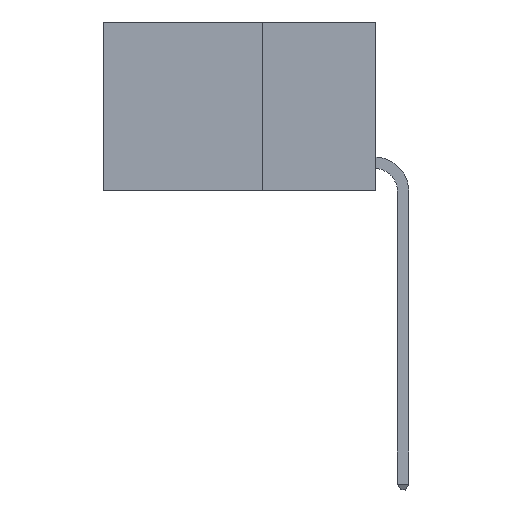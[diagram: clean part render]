
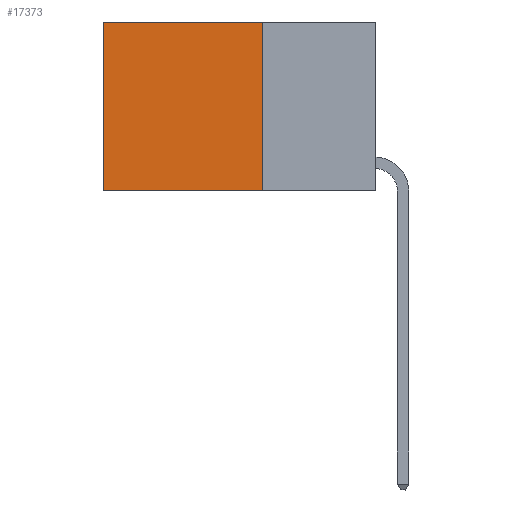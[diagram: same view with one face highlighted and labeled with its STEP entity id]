
A CAD part, left-side view. The second image highlights one B-rep face of the part: STEP entity #17373.
In plain terms, the highlighted planar face has unit normal (-1, 0, 0).
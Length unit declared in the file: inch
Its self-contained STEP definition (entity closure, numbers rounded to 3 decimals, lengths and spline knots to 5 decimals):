
#491 = LINE ( 'NONE', #16067, #17089 ) ;
#1017 = DIRECTION ( 'NONE',  ( 0., 1., 0. ) ) ;
#1060 = CARTESIAN_POINT ( 'NONE',  ( 0.2625, 0.25, 0. ) ) ;
#1243 = LINE ( 'NONE', #16291, #4562 ) ;
#3057 = CARTESIAN_POINT ( 'NONE',  ( 0.2625, 0.25, 0. ) ) ;
#3157 = EDGE_CURVE ( 'NONE', #7044, #5216, #16263, .T. ) ;
#4519 = VECTOR ( 'NONE', #12428, 39.37008 ) ;
#4562 = VECTOR ( 'NONE', #15044, 39.37008 ) ;
#5160 = CARTESIAN_POINT ( 'NONE',  ( 0.2625, 0.6, 0. ) ) ;
#5216 = VERTEX_POINT ( 'NONE', #5160 ) ;
#5340 = PLANE ( 'NONE',  #12170 ) ;
#5537 = ORIENTED_EDGE ( 'NONE', *, *, #12146, .T. ) ;
#6135 = VECTOR ( 'NONE', #1017, 39.37008 ) ;
#6690 = CARTESIAN_POINT ( 'NONE',  ( 0.2625, 0.25, 0. ) ) ;
#7044 = VERTEX_POINT ( 'NONE', #13022 ) ;
#8002 = DIRECTION ( 'NONE',  ( 1., 0., 0. ) ) ;
#9162 = CARTESIAN_POINT ( 'NONE',  ( 0.2625, 0.6, -0.37 ) ) ;
#9425 = DIRECTION ( 'NONE',  ( 0., 0., -1. ) ) ;
#9434 = EDGE_LOOP ( 'NONE', ( #5537, #16105, #17376, #15710 ) ) ;
#9750 = CARTESIAN_POINT ( 'NONE',  ( 0.2625, 0.25, -0.37 ) ) ;
#10584 = EDGE_CURVE ( 'NONE', #7044, #10585, #14710, .T. ) ;
#10585 = VERTEX_POINT ( 'NONE', #9750 ) ;
#11096 = FACE_OUTER_BOUND ( 'NONE', #9434, .T. ) ;
#12146 = EDGE_CURVE ( 'NONE', #5216, #13254, #491, .T. ) ;
#12170 = AXIS2_PLACEMENT_3D ( 'NONE', #6690, #8002, #17223 ) ;
#12428 = DIRECTION ( 'NONE',  ( 0., 0., -1. ) ) ;
#13022 = CARTESIAN_POINT ( 'NONE',  ( 0.2625, 0.25, 0. ) ) ;
#13254 = VERTEX_POINT ( 'NONE', #9162 ) ;
#14710 = LINE ( 'NONE', #3057, #4519 ) ;
#15044 = DIRECTION ( 'NONE',  ( 0., 1., 0. ) ) ;
#15392 = EDGE_CURVE ( 'NONE', #10585, #13254, #1243, .T. ) ;
#15710 = ORIENTED_EDGE ( 'NONE', *, *, #3157, .T. ) ;
#16067 = CARTESIAN_POINT ( 'NONE',  ( 0.2625, 0.6, 0. ) ) ;
#16105 = ORIENTED_EDGE ( 'NONE', *, *, #15392, .F. ) ;
#16263 = LINE ( 'NONE', #1060, #6135 ) ;
#16291 = CARTESIAN_POINT ( 'NONE',  ( 0.2625, 0.25, -0.37 ) ) ;
#17089 = VECTOR ( 'NONE', #9425, 39.37008 ) ;
#17223 = DIRECTION ( 'NONE',  ( 0., 0., -1. ) ) ;
#17373 = ADVANCED_FACE ( 'NONE', ( #11096 ), #5340, .F. ) ;
#17376 = ORIENTED_EDGE ( 'NONE', *, *, #10584, .F. ) ;
